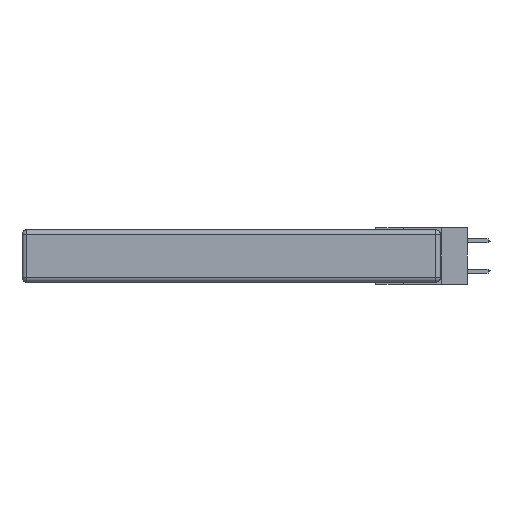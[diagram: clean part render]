
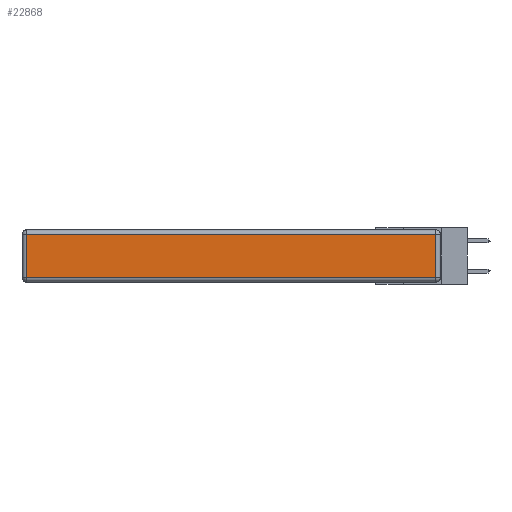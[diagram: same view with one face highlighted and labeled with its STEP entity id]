
A CAD part, left-side view. The second image highlights one B-rep face of the part: STEP entity #22868.
In plain terms, the highlighted planar face has unit normal (-1, 0, 0).
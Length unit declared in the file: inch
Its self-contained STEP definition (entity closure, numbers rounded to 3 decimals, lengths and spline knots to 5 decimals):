
#164 = AXIS2_PLACEMENT_3D ( 'NONE', #22987, #14173, #2707 ) ;
#1499 = CARTESIAN_POINT ( 'NONE',  ( 0., 0.03, -0.343 ) ) ;
#2449 = ORIENTED_EDGE ( 'NONE', *, *, #8470, .T. ) ;
#2707 = DIRECTION ( 'NONE',  ( 0., 0., 1. ) ) ;
#2766 = LINE ( 'NONE', #19012, #16861 ) ;
#5805 = VECTOR ( 'NONE', #14007, 39.37008 ) ;
#6803 = EDGE_CURVE ( 'NONE', #18171, #18628, #18946, .T. ) ;
#8002 = ORIENTED_EDGE ( 'NONE', *, *, #17671, .T. ) ;
#8470 = EDGE_CURVE ( 'NONE', #11664, #18171, #25836, .T. ) ;
#10061 = CARTESIAN_POINT ( 'NONE',  ( 0., 0., -0.313 ) ) ;
#10379 = CARTESIAN_POINT ( 'NONE',  ( 0., 0.03, -0.313 ) ) ;
#11664 = VERTEX_POINT ( 'NONE', #23156 ) ;
#12936 = VECTOR ( 'NONE', #19966, 39.37008 ) ;
#13890 = EDGE_CURVE ( 'NONE', #20086, #11664, #2766, .T. ) ;
#14007 = DIRECTION ( 'NONE',  ( 0., 0., -1. ) ) ;
#14173 = DIRECTION ( 'NONE',  ( -1., 0., 0. ) ) ;
#14485 = DIRECTION ( 'NONE',  ( 0., 1., 0. ) ) ;
#14690 = ORIENTED_EDGE ( 'NONE', *, *, #13890, .T. ) ;
#16170 = PLANE ( 'NONE',  #164 ) ;
#16861 = VECTOR ( 'NONE', #14485, 39.37008 ) ;
#17671 = EDGE_CURVE ( 'NONE', #18628, #20086, #28088, .T. ) ;
#17743 = CARTESIAN_POINT ( 'NONE',  ( 0., 0.03, -0.03 ) ) ;
#18165 = CARTESIAN_POINT ( 'NONE',  ( 0., 2.72, -0.343 ) ) ;
#18171 = VERTEX_POINT ( 'NONE', #27918 ) ;
#18628 = VERTEX_POINT ( 'NONE', #10379 ) ;
#18946 = LINE ( 'NONE', #10061, #12936 ) ;
#19012 = CARTESIAN_POINT ( 'NONE',  ( 0., 2.75, -0.03 ) ) ;
#19892 = EDGE_LOOP ( 'NONE', ( #22943, #8002, #14690, #2449 ) ) ;
#19966 = DIRECTION ( 'NONE',  ( 0., -1., 0. ) ) ;
#20086 = VERTEX_POINT ( 'NONE', #17743 ) ;
#21448 = VECTOR ( 'NONE', #23929, 39.37008 ) ;
#22868 = ADVANCED_FACE ( 'NONE', ( #26966 ), #16170, .T. ) ;
#22943 = ORIENTED_EDGE ( 'NONE', *, *, #6803, .T. ) ;
#22987 = CARTESIAN_POINT ( 'NONE',  ( 0., 0., -0.343 ) ) ;
#23156 = CARTESIAN_POINT ( 'NONE',  ( 0., 2.72, -0.03 ) ) ;
#23929 = DIRECTION ( 'NONE',  ( 0., 0., 1. ) ) ;
#25836 = LINE ( 'NONE', #18165, #5805 ) ;
#26966 = FACE_OUTER_BOUND ( 'NONE', #19892, .T. ) ;
#27918 = CARTESIAN_POINT ( 'NONE',  ( 0., 2.72, -0.313 ) ) ;
#28088 = LINE ( 'NONE', #1499, #21448 ) ;
